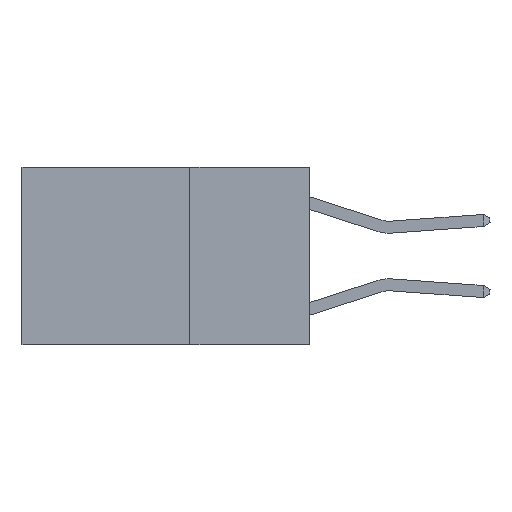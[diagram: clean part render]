
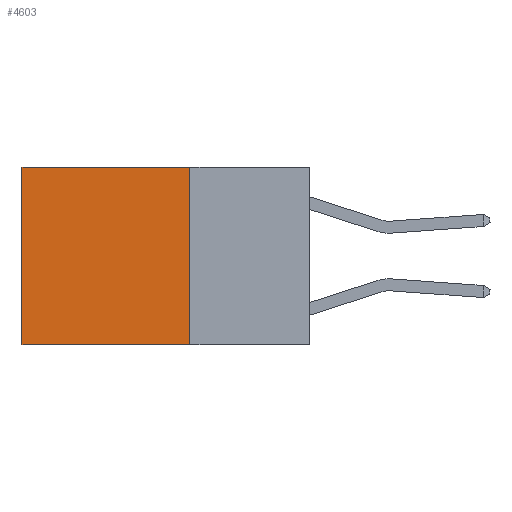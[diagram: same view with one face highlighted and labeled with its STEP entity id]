
A CAD part, left-side view. The second image highlights one B-rep face of the part: STEP entity #4603.
In plain terms, the highlighted planar face has unit normal (-1, 0, 0).
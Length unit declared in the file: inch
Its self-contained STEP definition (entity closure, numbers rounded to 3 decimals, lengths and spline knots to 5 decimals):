
#133 = PLANE ( 'NONE',  #9724 ) ;
#396 = CARTESIAN_POINT ( 'NONE',  ( 0.2625, 0.6, 0. ) ) ;
#734 = VECTOR ( 'NONE', #11682, 39.37008 ) ;
#2486 = ORIENTED_EDGE ( 'NONE', *, *, #14144, .F. ) ;
#3266 = CARTESIAN_POINT ( 'NONE',  ( 0.2625, 0.25, -0.37 ) ) ;
#3352 = DIRECTION ( 'NONE',  ( 0., 0., -1. ) ) ;
#3598 = DIRECTION ( 'NONE',  ( 1., 0., 0. ) ) ;
#3934 = LINE ( 'NONE', #9057, #13822 ) ;
#4212 = VERTEX_POINT ( 'NONE', #12861 ) ;
#4603 = ADVANCED_FACE ( 'NONE', ( #12924 ), #133, .F. ) ;
#4662 = VECTOR ( 'NONE', #11115, 39.37008 ) ;
#5196 = LINE ( 'NONE', #10347, #734 ) ;
#5885 = VERTEX_POINT ( 'NONE', #3266 ) ;
#5887 = CARTESIAN_POINT ( 'NONE',  ( 0.2625, 0.25, 0. ) ) ;
#6264 = DIRECTION ( 'NONE',  ( 0., 0., -1. ) ) ;
#6727 = ORIENTED_EDGE ( 'NONE', *, *, #16346, .T. ) ;
#9057 = CARTESIAN_POINT ( 'NONE',  ( 0.2625, 0.25, 0. ) ) ;
#9537 = LINE ( 'NONE', #396, #12543 ) ;
#9724 = AXIS2_PLACEMENT_3D ( 'NONE', #9976, #3598, #6264 ) ;
#9976 = CARTESIAN_POINT ( 'NONE',  ( 0.2625, 0.25, 0. ) ) ;
#10347 = CARTESIAN_POINT ( 'NONE',  ( 0.2625, 0.25, -0.37 ) ) ;
#10751 = ORIENTED_EDGE ( 'NONE', *, *, #12898, .T. ) ;
#11115 = DIRECTION ( 'NONE',  ( 0., 1., 0. ) ) ;
#11154 = CARTESIAN_POINT ( 'NONE',  ( 0.2625, 0.6, 0. ) ) ;
#11682 = DIRECTION ( 'NONE',  ( 0., 1., 0. ) ) ;
#12209 = ORIENTED_EDGE ( 'NONE', *, *, #13596, .F. ) ;
#12312 = LINE ( 'NONE', #5887, #4662 ) ;
#12543 = VECTOR ( 'NONE', #3352, 39.37008 ) ;
#12861 = CARTESIAN_POINT ( 'NONE',  ( 0.2625, 0.6, -0.37 ) ) ;
#12869 = EDGE_LOOP ( 'NONE', ( #10751, #12209, #2486, #6727 ) ) ;
#12898 = EDGE_CURVE ( 'NONE', #15401, #4212, #9537, .T. ) ;
#12901 = CARTESIAN_POINT ( 'NONE',  ( 0.2625, 0.25, 0. ) ) ;
#12924 = FACE_OUTER_BOUND ( 'NONE', #12869, .T. ) ;
#13596 = EDGE_CURVE ( 'NONE', #5885, #4212, #5196, .T. ) ;
#13822 = VECTOR ( 'NONE', #14608, 39.37008 ) ;
#14144 = EDGE_CURVE ( 'NONE', #16092, #5885, #3934, .T. ) ;
#14608 = DIRECTION ( 'NONE',  ( 0., 0., -1. ) ) ;
#15401 = VERTEX_POINT ( 'NONE', #11154 ) ;
#16092 = VERTEX_POINT ( 'NONE', #12901 ) ;
#16346 = EDGE_CURVE ( 'NONE', #16092, #15401, #12312, .T. ) ;
